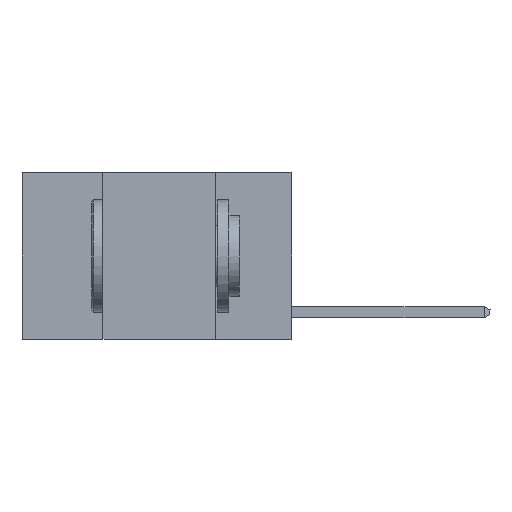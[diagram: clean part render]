
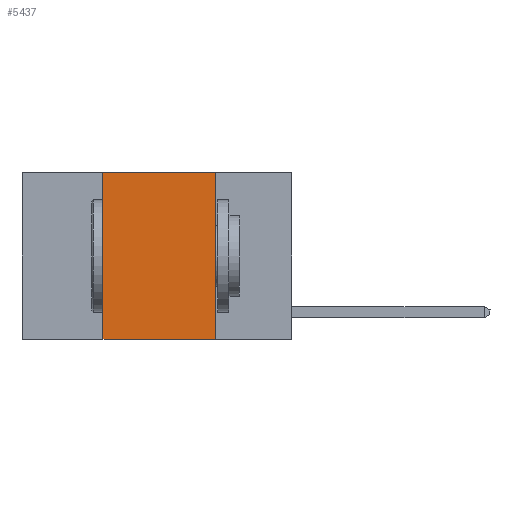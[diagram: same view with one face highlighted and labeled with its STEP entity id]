
A CAD part, left-side view. The second image highlights one B-rep face of the part: STEP entity #5437.
In plain terms, the highlighted planar face has unit normal (-1, 0, 0).
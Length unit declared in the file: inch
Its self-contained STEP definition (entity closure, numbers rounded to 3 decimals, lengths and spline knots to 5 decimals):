
#319 = VECTOR ( 'NONE', #9584, 39.37008 ) ;
#782 = VERTEX_POINT ( 'NONE', #6511 ) ;
#1204 = CARTESIAN_POINT ( 'NONE',  ( 0., 0.42, 0. ) ) ;
#1220 = AXIS2_PLACEMENT_3D ( 'NONE', #12787, #12090, #4078 ) ;
#1358 = VERTEX_POINT ( 'NONE', #10806 ) ;
#2283 = EDGE_CURVE ( 'NONE', #14374, #1358, #9118, .T. ) ;
#2741 = CARTESIAN_POINT ( 'NONE',  ( 0., 0.6, 0. ) ) ;
#3339 = LINE ( 'NONE', #1204, #319 ) ;
#4078 = DIRECTION ( 'NONE',  ( 0., 0., -1. ) ) ;
#4877 = LINE ( 'NONE', #6254, #13181 ) ;
#5437 = ADVANCED_FACE ( 'NONE', ( #6213 ), #10259, .F. ) ;
#6213 = FACE_OUTER_BOUND ( 'NONE', #12259, .T. ) ;
#6239 = DIRECTION ( 'NONE',  ( 0., -1., 0. ) ) ;
#6254 = CARTESIAN_POINT ( 'NONE',  ( 0., 0.6, -0.37 ) ) ;
#6511 = CARTESIAN_POINT ( 'NONE',  ( 0., 0.42, 0. ) ) ;
#6586 = DIRECTION ( 'NONE',  ( 0., 0., -1. ) ) ;
#7479 = DIRECTION ( 'NONE',  ( 0., -1., 0. ) ) ;
#9118 = LINE ( 'NONE', #12588, #15201 ) ;
#9516 = ORIENTED_EDGE ( 'NONE', *, *, #15288, .F. ) ;
#9584 = DIRECTION ( 'NONE',  ( 0., 0., 1. ) ) ;
#9899 = CARTESIAN_POINT ( 'NONE',  ( 0., 0.42, -0.37 ) ) ;
#10259 = PLANE ( 'NONE',  #1220 ) ;
#10806 = CARTESIAN_POINT ( 'NONE',  ( 0., 0.17, -0.37 ) ) ;
#10973 = VECTOR ( 'NONE', #6239, 39.37008 ) ;
#11211 = EDGE_CURVE ( 'NONE', #782, #14374, #12855, .T. ) ;
#11810 = VERTEX_POINT ( 'NONE', #9899 ) ;
#12090 = DIRECTION ( 'NONE',  ( 1., 0., 0. ) ) ;
#12259 = EDGE_LOOP ( 'NONE', ( #15662, #15338, #9516, #15326 ) ) ;
#12588 = CARTESIAN_POINT ( 'NONE',  ( 0., 0.17, 0. ) ) ;
#12787 = CARTESIAN_POINT ( 'NONE',  ( 0., 0.6, 0. ) ) ;
#12855 = LINE ( 'NONE', #2741, #10973 ) ;
#13181 = VECTOR ( 'NONE', #7479, 39.37008 ) ;
#14374 = VERTEX_POINT ( 'NONE', #14853 ) ;
#14853 = CARTESIAN_POINT ( 'NONE',  ( 0., 0.17, 0. ) ) ;
#15201 = VECTOR ( 'NONE', #6586, 39.37008 ) ;
#15288 = EDGE_CURVE ( 'NONE', #11810, #782, #3339, .T. ) ;
#15326 = ORIENTED_EDGE ( 'NONE', *, *, #15603, .T. ) ;
#15338 = ORIENTED_EDGE ( 'NONE', *, *, #11211, .F. ) ;
#15603 = EDGE_CURVE ( 'NONE', #11810, #1358, #4877, .T. ) ;
#15662 = ORIENTED_EDGE ( 'NONE', *, *, #2283, .F. ) ;
